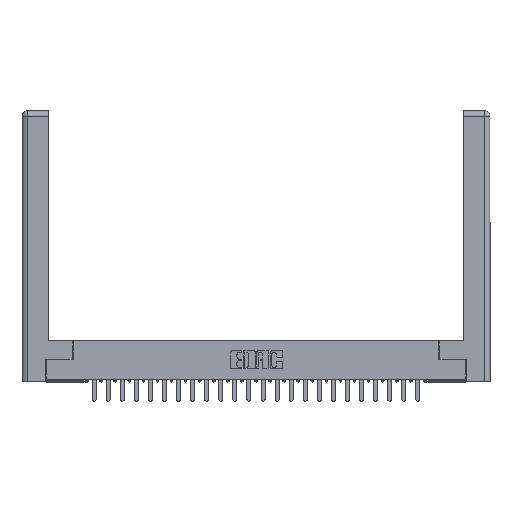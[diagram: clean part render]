
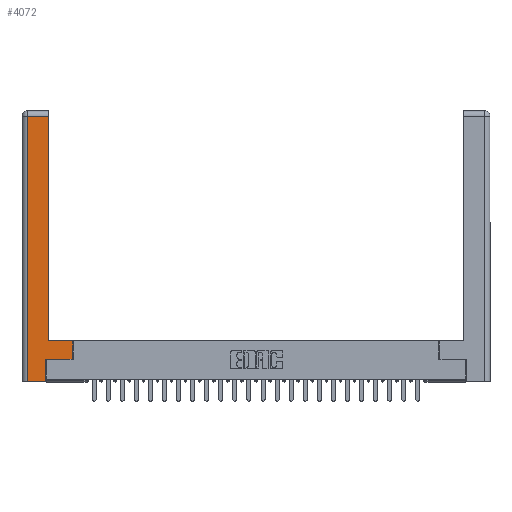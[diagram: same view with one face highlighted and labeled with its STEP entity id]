
A CAD part, top view. The second image highlights one B-rep face of the part: STEP entity #4072.
In plain terms, the highlighted planar face has unit normal (0, 0, 1).
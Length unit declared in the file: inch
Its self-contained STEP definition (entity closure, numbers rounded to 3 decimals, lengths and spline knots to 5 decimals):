
#123 = LINE ( 'NONE', #2918, #11199 ) ;
#461 = VECTOR ( 'NONE', #1193, 39.37008 ) ;
#466 = VERTEX_POINT ( 'NONE', #2176 ) ;
#800 = DIRECTION ( 'NONE',  ( -1., 0., 0. ) ) ;
#805 = CARTESIAN_POINT ( 'NONE',  ( 0.265, 0.245, 0. ) ) ;
#1193 = DIRECTION ( 'NONE',  ( 0., 1., 0. ) ) ;
#1196 = DIRECTION ( 'NONE',  ( 0., 1., 0. ) ) ;
#1539 = ORIENTED_EDGE ( 'NONE', *, *, #5510, .T. ) ;
#1868 = DIRECTION ( 'NONE',  ( 1., 0., 0. ) ) ;
#2118 = VECTOR ( 'NONE', #29140, 39.37008 ) ;
#2176 = CARTESIAN_POINT ( 'NONE',  ( 0.0615, 2.94, 0. ) ) ;
#2355 = EDGE_CURVE ( 'NONE', #13140, #466, #4054, .T. ) ;
#2644 = ORIENTED_EDGE ( 'NONE', *, *, #2355, .T. ) ;
#2918 = CARTESIAN_POINT ( 'NONE',  ( 0.295, 0.45, 0. ) ) ;
#2977 = ORIENTED_EDGE ( 'NONE', *, *, #21545, .T. ) ;
#4029 = CARTESIAN_POINT ( 'NONE',  ( 0.295, 2.94, 0. ) ) ;
#4054 = LINE ( 'NONE', #20011, #19596 ) ;
#4072 = ADVANCED_FACE ( 'NONE', ( #17610 ), #20109, .F. ) ;
#5510 = EDGE_CURVE ( 'NONE', #12174, #20067, #30355, .T. ) ;
#5637 = DIRECTION ( 'NONE',  ( 1., 0., 0. ) ) ;
#5947 = CARTESIAN_POINT ( 'NONE',  ( 0., 0., 0. ) ) ;
#8894 = CARTESIAN_POINT ( 'NONE',  ( 0.265, 0., 0. ) ) ;
#9383 = CARTESIAN_POINT ( 'NONE',  ( 0.265, 0.245, 0. ) ) ;
#9581 = LINE ( 'NONE', #8894, #12882 ) ;
#10299 = CARTESIAN_POINT ( 'NONE',  ( 0.565, 0.245, 0. ) ) ;
#11199 = VECTOR ( 'NONE', #15490, 39.37008 ) ;
#12174 = VERTEX_POINT ( 'NONE', #9383 ) ;
#12218 = VECTOR ( 'NONE', #25506, 39.37008 ) ;
#12882 = VECTOR ( 'NONE', #1868, 39.37008 ) ;
#13028 = ORIENTED_EDGE ( 'NONE', *, *, #24303, .T. ) ;
#13140 = VERTEX_POINT ( 'NONE', #4029 ) ;
#13413 = CARTESIAN_POINT ( 'NONE',  ( 0.265, 0., 0. ) ) ;
#13521 = CARTESIAN_POINT ( 'NONE',  ( 0.565, 0.245, 0. ) ) ;
#13586 = LINE ( 'NONE', #26802, #2118 ) ;
#14211 = EDGE_CURVE ( 'NONE', #17003, #16774, #123, .T. ) ;
#14892 = AXIS2_PLACEMENT_3D ( 'NONE', #5947, #22533, #17944 ) ;
#15014 = ORIENTED_EDGE ( 'NONE', *, *, #29540, .T. ) ;
#15144 = VECTOR ( 'NONE', #1196, 39.37008 ) ;
#15255 = CARTESIAN_POINT ( 'NONE',  ( 0.295, 0.45, 0. ) ) ;
#15490 = DIRECTION ( 'NONE',  ( -1., 0., 0. ) ) ;
#15863 = CARTESIAN_POINT ( 'NONE',  ( 0.295, 3., 0. ) ) ;
#16774 = VERTEX_POINT ( 'NONE', #15255 ) ;
#16869 = EDGE_CURVE ( 'NONE', #16774, #13140, #19987, .T. ) ;
#17003 = VERTEX_POINT ( 'NONE', #17413 ) ;
#17413 = CARTESIAN_POINT ( 'NONE',  ( 0.565, 0.45, 0. ) ) ;
#17610 = FACE_OUTER_BOUND ( 'NONE', #26866, .T. ) ;
#17944 = DIRECTION ( 'NONE',  ( -1., 0., 0. ) ) ;
#19596 = VECTOR ( 'NONE', #800, 39.37008 ) ;
#19910 = VECTOR ( 'NONE', #5637, 39.37008 ) ;
#19987 = LINE ( 'NONE', #15863, #12218 ) ;
#20011 = CARTESIAN_POINT ( 'NONE',  ( 0.0615, 2.94, 0. ) ) ;
#20067 = VERTEX_POINT ( 'NONE', #13521 ) ;
#20101 = VERTEX_POINT ( 'NONE', #13413 ) ;
#20109 = PLANE ( 'NONE',  #14892 ) ;
#21115 = LINE ( 'NONE', #27344, #15144 ) ;
#21545 = EDGE_CURVE ( 'NONE', #20101, #12174, #28269, .T. ) ;
#21552 = CARTESIAN_POINT ( 'NONE',  ( 0.0615, 0., 0. ) ) ;
#22359 = EDGE_CURVE ( 'NONE', #20067, #17003, #21115, .T. ) ;
#22533 = DIRECTION ( 'NONE',  ( 0., 0., -1. ) ) ;
#23034 = VERTEX_POINT ( 'NONE', #21552 ) ;
#23229 = ORIENTED_EDGE ( 'NONE', *, *, #16869, .T. ) ;
#24303 = EDGE_CURVE ( 'NONE', #466, #23034, #13586, .T. ) ;
#25506 = DIRECTION ( 'NONE',  ( 0., 1., 0. ) ) ;
#26620 = ORIENTED_EDGE ( 'NONE', *, *, #22359, .T. ) ;
#26802 = CARTESIAN_POINT ( 'NONE',  ( 0.0615, 0., 0. ) ) ;
#26866 = EDGE_LOOP ( 'NONE', ( #23229, #2644, #13028, #15014, #2977, #1539, #26620, #29804 ) ) ;
#27344 = CARTESIAN_POINT ( 'NONE',  ( 0.565, 0.45, 0. ) ) ;
#28269 = LINE ( 'NONE', #805, #461 ) ;
#29140 = DIRECTION ( 'NONE',  ( 0., -1., 0. ) ) ;
#29540 = EDGE_CURVE ( 'NONE', #23034, #20101, #9581, .T. ) ;
#29804 = ORIENTED_EDGE ( 'NONE', *, *, #14211, .T. ) ;
#30355 = LINE ( 'NONE', #10299, #19910 ) ;
